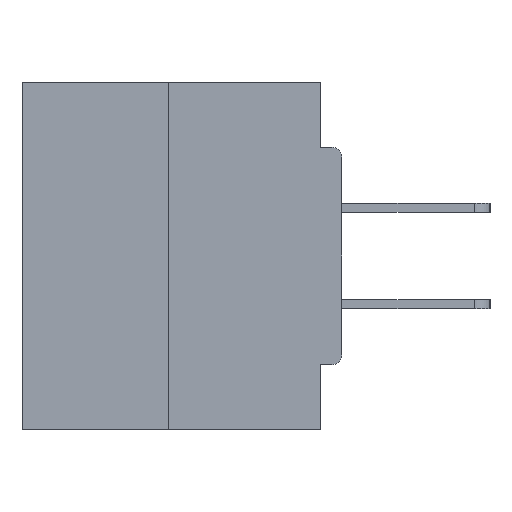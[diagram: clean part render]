
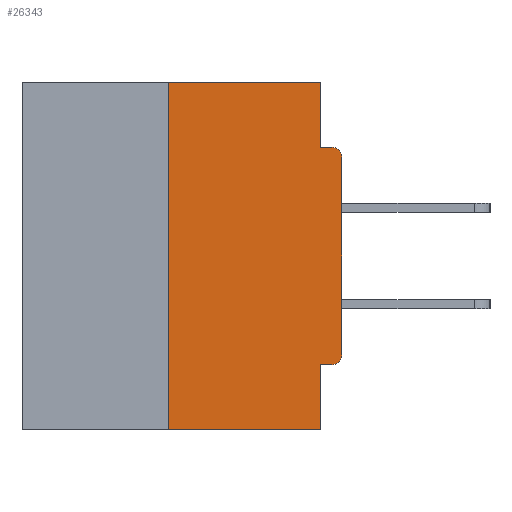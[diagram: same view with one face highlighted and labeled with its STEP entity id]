
A CAD part, left-side view. The second image highlights one B-rep face of the part: STEP entity #26343.
In plain terms, the highlighted planar face has unit normal (-1, 0, 0).
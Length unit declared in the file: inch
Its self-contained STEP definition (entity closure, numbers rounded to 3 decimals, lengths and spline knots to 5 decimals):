
#262 = PLANE ( 'NONE',  #673 ) ;
#405 = VERTEX_POINT ( 'NONE', #26125 ) ;
#673 = AXIS2_PLACEMENT_3D ( 'NONE', #19333, #8360, #2924 ) ;
#1070 = CIRCLE ( 'NONE', #29943, 0.015 ) ;
#1297 = CARTESIAN_POINT ( 'NONE',  ( 0., 0., -0.1085 ) ) ;
#1689 = AXIS2_PLACEMENT_3D ( 'NONE', #19315, #24474, #30415 ) ;
#2924 = DIRECTION ( 'NONE',  ( 0., 0., -1. ) ) ;
#4025 = ORIENTED_EDGE ( 'NONE', *, *, #32175, .F. ) ;
#4289 = ORIENTED_EDGE ( 'NONE', *, *, #33450, .F. ) ;
#5006 = DIRECTION ( 'NONE',  ( 0., 0., -1. ) ) ;
#5029 = DIRECTION ( 'NONE',  ( 0., 0., 1. ) ) ;
#5147 = CARTESIAN_POINT ( 'NONE',  ( 0., 0., -0.3915 ) ) ;
#5213 = CARTESIAN_POINT ( 'NONE',  ( 0., 0.031, 0. ) ) ;
#5619 = VECTOR ( 'NONE', #26784, 39.37008 ) ;
#6743 = ORIENTED_EDGE ( 'NONE', *, *, #16416, .F. ) ;
#7253 = CARTESIAN_POINT ( 'NONE',  ( 0., 0.015, -0.4065 ) ) ;
#7491 = CARTESIAN_POINT ( 'NONE',  ( 0., 0.031, -0.4065 ) ) ;
#7758 = CARTESIAN_POINT ( 'NONE',  ( 0., 0.031, 0. ) ) ;
#8360 = DIRECTION ( 'NONE',  ( 1., 0., 0. ) ) ;
#8508 = CARTESIAN_POINT ( 'NONE',  ( 0., 0., -0.0935 ) ) ;
#8602 = CARTESIAN_POINT ( 'NONE',  ( 0., 0.015, -0.0935 ) ) ;
#9734 = VECTOR ( 'NONE', #29857, 39.37008 ) ;
#11176 = VECTOR ( 'NONE', #29674, 39.37008 ) ;
#11675 = CARTESIAN_POINT ( 'NONE',  ( 0., 0.015, -0.3915 ) ) ;
#12358 = LINE ( 'NONE', #5213, #26984 ) ;
#13251 = CARTESIAN_POINT ( 'NONE',  ( 0., 0.031, -0.5 ) ) ;
#13762 = EDGE_CURVE ( 'NONE', #30027, #28756, #1070, .T. ) ;
#14520 = DIRECTION ( 'NONE',  ( 0., -1., 0. ) ) ;
#15189 = EDGE_LOOP ( 'NONE', ( #6743, #4289, #16903, #30859, #28184, #27255, #25782, #19751, #25986, #4025 ) ) ;
#16416 = EDGE_CURVE ( 'NONE', #405, #31348, #25025, .T. ) ;
#16903 = ORIENTED_EDGE ( 'NONE', *, *, #27700, .T. ) ;
#17096 = CARTESIAN_POINT ( 'NONE',  ( 0., 0.25, -0.5 ) ) ;
#17250 = DIRECTION ( 'NONE',  ( -1., 0., 0. ) ) ;
#17333 = EDGE_CURVE ( 'NONE', #30027, #26134, #22362, .T. ) ;
#17945 = CARTESIAN_POINT ( 'NONE',  ( 0., 0.031, -0.0935 ) ) ;
#19315 = CARTESIAN_POINT ( 'NONE',  ( 0., 0.015, -0.1085 ) ) ;
#19333 = CARTESIAN_POINT ( 'NONE',  ( 0., 0.46, 0. ) ) ;
#19751 = ORIENTED_EDGE ( 'NONE', *, *, #23249, .T. ) ;
#20030 = FACE_OUTER_BOUND ( 'NONE', #15189, .T. ) ;
#20031 = VECTOR ( 'NONE', #14520, 39.37008 ) ;
#20853 = VERTEX_POINT ( 'NONE', #22953 ) ;
#21051 = CARTESIAN_POINT ( 'NONE',  ( 0., 0.46, -0.5 ) ) ;
#22158 = EDGE_CURVE ( 'NONE', #26134, #20853, #26779, .T. ) ;
#22362 = LINE ( 'NONE', #24462, #11176 ) ;
#22586 = VERTEX_POINT ( 'NONE', #17945 ) ;
#22889 = VECTOR ( 'NONE', #5029, 39.37008 ) ;
#22913 = VECTOR ( 'NONE', #23594, 39.37008 ) ;
#22953 = CARTESIAN_POINT ( 'NONE',  ( 0., 0.031, -0.5 ) ) ;
#23249 = EDGE_CURVE ( 'NONE', #35039, #26355, #25385, .T. ) ;
#23594 = DIRECTION ( 'NONE',  ( 0., -1., 0. ) ) ;
#24462 = CARTESIAN_POINT ( 'NONE',  ( 0., 0., -0.4065 ) ) ;
#24474 = DIRECTION ( 'NONE',  ( -1., 0., 0. ) ) ;
#24600 = VECTOR ( 'NONE', #5006, 39.37008 ) ;
#24997 = VERTEX_POINT ( 'NONE', #17096 ) ;
#25025 = LINE ( 'NONE', #32606, #5619 ) ;
#25230 = LINE ( 'NONE', #35047, #9734 ) ;
#25385 = CIRCLE ( 'NONE', #1689, 0.015 ) ;
#25782 = ORIENTED_EDGE ( 'NONE', *, *, #28758, .T. ) ;
#25986 = ORIENTED_EDGE ( 'NONE', *, *, #33687, .F. ) ;
#26125 = CARTESIAN_POINT ( 'NONE',  ( 0., 0.25, 0. ) ) ;
#26134 = VERTEX_POINT ( 'NONE', #7491 ) ;
#26343 = ADVANCED_FACE ( 'NONE', ( #20030 ), #262, .F. ) ;
#26355 = VERTEX_POINT ( 'NONE', #8602 ) ;
#26779 = LINE ( 'NONE', #13251, #24600 ) ;
#26784 = DIRECTION ( 'NONE',  ( 0., -1., 0. ) ) ;
#26984 = VECTOR ( 'NONE', #35608, 39.37008 ) ;
#27200 = CARTESIAN_POINT ( 'NONE',  ( 0., 0., 0. ) ) ;
#27255 = ORIENTED_EDGE ( 'NONE', *, *, #13762, .T. ) ;
#27700 = EDGE_CURVE ( 'NONE', #24997, #20853, #29409, .T. ) ;
#28184 = ORIENTED_EDGE ( 'NONE', *, *, #17333, .F. ) ;
#28756 = VERTEX_POINT ( 'NONE', #5147 ) ;
#28758 = EDGE_CURVE ( 'NONE', #28756, #35039, #32867, .T. ) ;
#29409 = LINE ( 'NONE', #21051, #22913 ) ;
#29674 = DIRECTION ( 'NONE',  ( 0., 1., 0. ) ) ;
#29857 = DIRECTION ( 'NONE',  ( 0., 0., 1. ) ) ;
#29943 = AXIS2_PLACEMENT_3D ( 'NONE', #11675, #17250, #30987 ) ;
#30027 = VERTEX_POINT ( 'NONE', #7253 ) ;
#30415 = DIRECTION ( 'NONE',  ( 0., 0., -1. ) ) ;
#30859 = ORIENTED_EDGE ( 'NONE', *, *, #22158, .F. ) ;
#30987 = DIRECTION ( 'NONE',  ( 0., 0., -1. ) ) ;
#31348 = VERTEX_POINT ( 'NONE', #7758 ) ;
#32175 = EDGE_CURVE ( 'NONE', #31348, #22586, #12358, .T. ) ;
#32606 = CARTESIAN_POINT ( 'NONE',  ( 0., 0.46, 0. ) ) ;
#32867 = LINE ( 'NONE', #27200, #22889 ) ;
#33450 = EDGE_CURVE ( 'NONE', #24997, #405, #25230, .T. ) ;
#33687 = EDGE_CURVE ( 'NONE', #22586, #26355, #33853, .T. ) ;
#33853 = LINE ( 'NONE', #8508, #20031 ) ;
#35039 = VERTEX_POINT ( 'NONE', #1297 ) ;
#35047 = CARTESIAN_POINT ( 'NONE',  ( 0., 0.25, 0. ) ) ;
#35608 = DIRECTION ( 'NONE',  ( 0., 0., -1. ) ) ;
